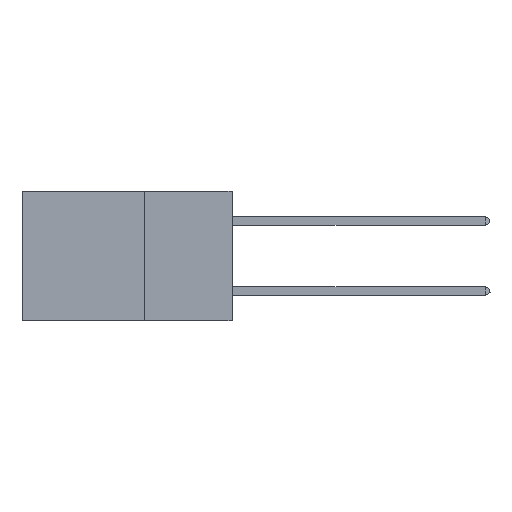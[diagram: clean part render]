
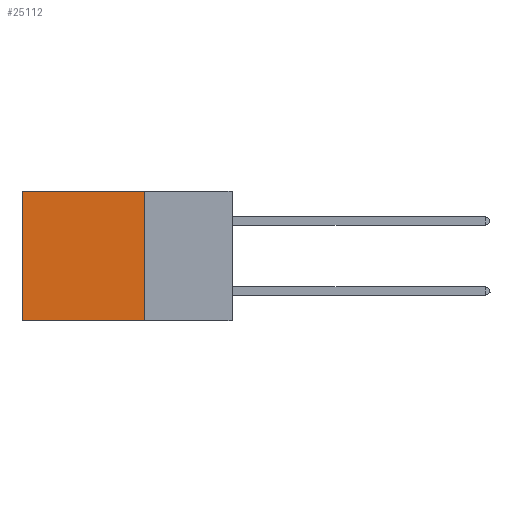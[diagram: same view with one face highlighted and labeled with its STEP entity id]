
A CAD part, left-side view. The second image highlights one B-rep face of the part: STEP entity #25112.
In plain terms, the highlighted planar face has unit normal (-1, 0, 0).
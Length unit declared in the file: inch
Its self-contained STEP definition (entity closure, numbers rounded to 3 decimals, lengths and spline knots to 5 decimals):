
#248 = DIRECTION ( 'NONE',  ( 0., 0., -1. ) ) ;
#323 = LINE ( 'NONE', #17990, #6396 ) ;
#758 = ORIENTED_EDGE ( 'NONE', *, *, #21814, .F. ) ;
#1818 = VECTOR ( 'NONE', #44083, 39.37008 ) ;
#4907 = ORIENTED_EDGE ( 'NONE', *, *, #25551, .F. ) ;
#5506 = AXIS2_PLACEMENT_3D ( 'NONE', #17081, #45249, #10239 ) ;
#6231 = LINE ( 'NONE', #26292, #1818 ) ;
#6396 = VECTOR ( 'NONE', #29253, 39.37008 ) ;
#9240 = VECTOR ( 'NONE', #15964, 39.37008 ) ;
#10239 = DIRECTION ( 'NONE',  ( 0., 0., -1. ) ) ;
#11956 = ORIENTED_EDGE ( 'NONE', *, *, #13750, .T. ) ;
#13750 = EDGE_CURVE ( 'NONE', #31821, #15610, #18432, .T. ) ;
#15610 = VERTEX_POINT ( 'NONE', #37531 ) ;
#15964 = DIRECTION ( 'NONE',  ( 0., 1., 0. ) ) ;
#16928 = VERTEX_POINT ( 'NONE', #24119 ) ;
#17081 = CARTESIAN_POINT ( 'NONE',  ( 0.2875, 0.25, 0. ) ) ;
#17990 = CARTESIAN_POINT ( 'NONE',  ( 0.2875, 0.25, 0. ) ) ;
#18432 = LINE ( 'NONE', #43408, #28375 ) ;
#18547 = EDGE_CURVE ( 'NONE', #43530, #31821, #323, .T. ) ;
#21814 = EDGE_CURVE ( 'NONE', #43530, #16928, #6231, .T. ) ;
#24119 = CARTESIAN_POINT ( 'NONE',  ( 0.2875, 0.25, -0.37 ) ) ;
#24647 = PLANE ( 'NONE',  #5506 ) ;
#25112 = ADVANCED_FACE ( 'NONE', ( #38639 ), #24647, .F. ) ;
#25551 = EDGE_CURVE ( 'NONE', #16928, #15610, #27490, .T. ) ;
#26292 = CARTESIAN_POINT ( 'NONE',  ( 0.2875, 0.25, 0. ) ) ;
#27490 = LINE ( 'NONE', #30315, #9240 ) ;
#28375 = VECTOR ( 'NONE', #248, 39.37008 ) ;
#29253 = DIRECTION ( 'NONE',  ( 0., 1., 0. ) ) ;
#30315 = CARTESIAN_POINT ( 'NONE',  ( 0.2875, 0.25, -0.37 ) ) ;
#31238 = ORIENTED_EDGE ( 'NONE', *, *, #18547, .T. ) ;
#31821 = VERTEX_POINT ( 'NONE', #39250 ) ;
#37531 = CARTESIAN_POINT ( 'NONE',  ( 0.2875, 0.6, -0.37 ) ) ;
#38639 = FACE_OUTER_BOUND ( 'NONE', #45657, .T. ) ;
#39250 = CARTESIAN_POINT ( 'NONE',  ( 0.2875, 0.6, 0. ) ) ;
#40181 = CARTESIAN_POINT ( 'NONE',  ( 0.2875, 0.25, 0. ) ) ;
#43408 = CARTESIAN_POINT ( 'NONE',  ( 0.2875, 0.6, 0. ) ) ;
#43530 = VERTEX_POINT ( 'NONE', #40181 ) ;
#44083 = DIRECTION ( 'NONE',  ( 0., 0., -1. ) ) ;
#45249 = DIRECTION ( 'NONE',  ( 1., 0., 0. ) ) ;
#45657 = EDGE_LOOP ( 'NONE', ( #11956, #4907, #758, #31238 ) ) ;
